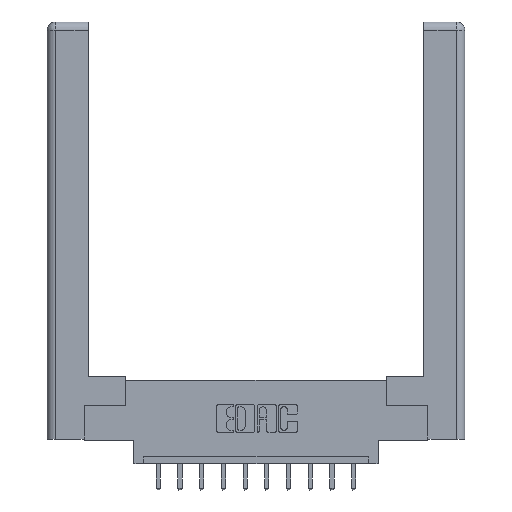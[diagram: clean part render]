
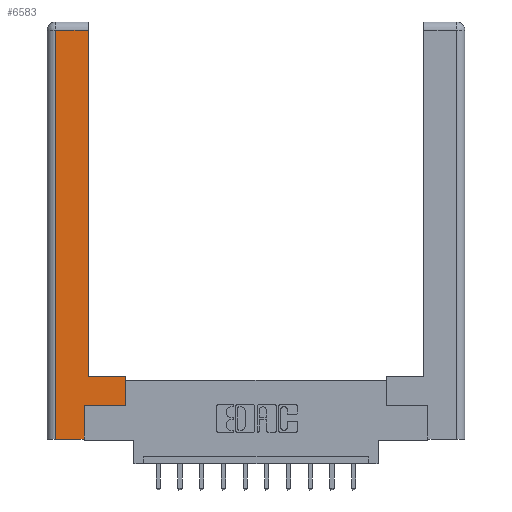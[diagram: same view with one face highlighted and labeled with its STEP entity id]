
A CAD part, top view. The second image highlights one B-rep face of the part: STEP entity #6583.
In plain terms, the highlighted planar face has unit normal (0, 0, 1).
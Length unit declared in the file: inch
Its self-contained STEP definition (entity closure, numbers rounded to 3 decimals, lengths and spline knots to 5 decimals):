
#58 = EDGE_CURVE ( 'NONE', #14129, #3923, #4173, .T. ) ;
#433 = CARTESIAN_POINT ( 'NONE',  ( 0.265, 0.245, 0. ) ) ;
#505 = DIRECTION ( 'NONE',  ( 1., 0., 0. ) ) ;
#662 = CARTESIAN_POINT ( 'NONE',  ( 0.565, 0.245, 0. ) ) ;
#822 = VECTOR ( 'NONE', #8416, 39.37008 ) ;
#1211 = ORIENTED_EDGE ( 'NONE', *, *, #7550, .T. ) ;
#1260 = EDGE_LOOP ( 'NONE', ( #4792, #12861, #1211, #1395, #4387, #6333, #5866, #13499 ) ) ;
#1272 = EDGE_CURVE ( 'NONE', #2139, #4141, #2905, .T. ) ;
#1395 = ORIENTED_EDGE ( 'NONE', *, *, #58, .T. ) ;
#2139 = VERTEX_POINT ( 'NONE', #11822 ) ;
#2396 = CARTESIAN_POINT ( 'NONE',  ( 0.295, 0.45, 0. ) ) ;
#2465 = CARTESIAN_POINT ( 'NONE',  ( 0.265, 0., 0. ) ) ;
#2729 = LINE ( 'NONE', #7545, #13422 ) ;
#2836 = CARTESIAN_POINT ( 'NONE',  ( 0.265, 0., 0. ) ) ;
#2905 = LINE ( 'NONE', #4930, #14444 ) ;
#3923 = VERTEX_POINT ( 'NONE', #2836 ) ;
#3962 = CARTESIAN_POINT ( 'NONE',  ( 0.565, 0.45, 0. ) ) ;
#4141 = VERTEX_POINT ( 'NONE', #4289 ) ;
#4173 = LINE ( 'NONE', #2465, #14101 ) ;
#4289 = CARTESIAN_POINT ( 'NONE',  ( 0.0615, 2.94, 0. ) ) ;
#4387 = ORIENTED_EDGE ( 'NONE', *, *, #9098, .T. ) ;
#4792 = ORIENTED_EDGE ( 'NONE', *, *, #10007, .T. ) ;
#4881 = DIRECTION ( 'NONE',  ( -1., 0., 0. ) ) ;
#4930 = CARTESIAN_POINT ( 'NONE',  ( 0.0615, 2.94, 0. ) ) ;
#4954 = VERTEX_POINT ( 'NONE', #433 ) ;
#5368 = VERTEX_POINT ( 'NONE', #2396 ) ;
#5472 = EDGE_CURVE ( 'NONE', #6192, #5368, #13863, .T. ) ;
#5677 = LINE ( 'NONE', #11757, #13373 ) ;
#5848 = CARTESIAN_POINT ( 'NONE',  ( 0.565, 0.45, 0. ) ) ;
#5866 = ORIENTED_EDGE ( 'NONE', *, *, #9362, .T. ) ;
#5917 = CARTESIAN_POINT ( 'NONE',  ( 0., 0., 0. ) ) ;
#6192 = VERTEX_POINT ( 'NONE', #3962 ) ;
#6333 = ORIENTED_EDGE ( 'NONE', *, *, #10602, .T. ) ;
#6583 = ADVANCED_FACE ( 'NONE', ( #11582 ), #8096, .F. ) ;
#6840 = DIRECTION ( 'NONE',  ( -1., 0., 0. ) ) ;
#6995 = LINE ( 'NONE', #9651, #7505 ) ;
#7505 = VECTOR ( 'NONE', #13171, 39.37008 ) ;
#7545 = CARTESIAN_POINT ( 'NONE',  ( 0.265, 0.245, 0. ) ) ;
#7550 = EDGE_CURVE ( 'NONE', #4141, #14129, #6995, .T. ) ;
#7955 = DIRECTION ( 'NONE',  ( -1., 0., 0. ) ) ;
#8096 = PLANE ( 'NONE',  #13549 ) ;
#8416 = DIRECTION ( 'NONE',  ( 0., 1., 0. ) ) ;
#8659 = LINE ( 'NONE', #5848, #822 ) ;
#9098 = EDGE_CURVE ( 'NONE', #3923, #4954, #2729, .T. ) ;
#9362 = EDGE_CURVE ( 'NONE', #12343, #6192, #8659, .T. ) ;
#9651 = CARTESIAN_POINT ( 'NONE',  ( 0.0615, 0., 0. ) ) ;
#9950 = DIRECTION ( 'NONE',  ( 0., 1., 0. ) ) ;
#10007 = EDGE_CURVE ( 'NONE', #5368, #2139, #5677, .T. ) ;
#10120 = CARTESIAN_POINT ( 'NONE',  ( 0.295, 0.45, 0. ) ) ;
#10287 = VECTOR ( 'NONE', #505, 39.37008 ) ;
#10602 = EDGE_CURVE ( 'NONE', #4954, #12343, #14310, .T. ) ;
#10891 = VECTOR ( 'NONE', #7955, 39.37008 ) ;
#11582 = FACE_OUTER_BOUND ( 'NONE', #1260, .T. ) ;
#11757 = CARTESIAN_POINT ( 'NONE',  ( 0.295, 3., 0. ) ) ;
#11800 = DIRECTION ( 'NONE',  ( 0., 1., 0. ) ) ;
#11822 = CARTESIAN_POINT ( 'NONE',  ( 0.295, 2.94, 0. ) ) ;
#12343 = VERTEX_POINT ( 'NONE', #662 ) ;
#12509 = DIRECTION ( 'NONE',  ( 1., 0., 0. ) ) ;
#12521 = CARTESIAN_POINT ( 'NONE',  ( 0.0615, 0., 0. ) ) ;
#12712 = CARTESIAN_POINT ( 'NONE',  ( 0.565, 0.245, 0. ) ) ;
#12861 = ORIENTED_EDGE ( 'NONE', *, *, #1272, .T. ) ;
#13171 = DIRECTION ( 'NONE',  ( 0., -1., 0. ) ) ;
#13373 = VECTOR ( 'NONE', #11800, 39.37008 ) ;
#13422 = VECTOR ( 'NONE', #9950, 39.37008 ) ;
#13499 = ORIENTED_EDGE ( 'NONE', *, *, #5472, .T. ) ;
#13549 = AXIS2_PLACEMENT_3D ( 'NONE', #5917, #13731, #6840 ) ;
#13731 = DIRECTION ( 'NONE',  ( 0., 0., -1. ) ) ;
#13863 = LINE ( 'NONE', #10120, #10891 ) ;
#14101 = VECTOR ( 'NONE', #12509, 39.37008 ) ;
#14129 = VERTEX_POINT ( 'NONE', #12521 ) ;
#14310 = LINE ( 'NONE', #12712, #10287 ) ;
#14444 = VECTOR ( 'NONE', #4881, 39.37008 ) ;
